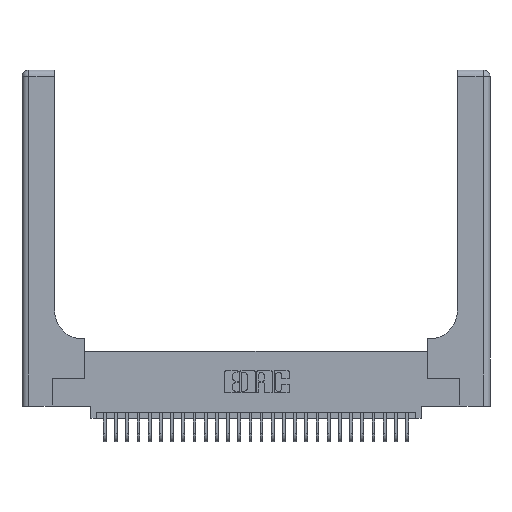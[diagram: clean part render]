
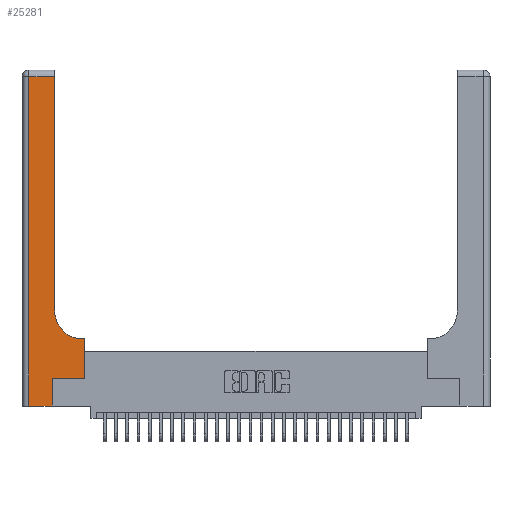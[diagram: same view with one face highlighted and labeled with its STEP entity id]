
A CAD part, top view. The second image highlights one B-rep face of the part: STEP entity #25281.
In plain terms, the highlighted planar face has unit normal (0, 0, 1).
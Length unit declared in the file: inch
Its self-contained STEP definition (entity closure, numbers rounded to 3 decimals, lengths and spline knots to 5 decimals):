
#190 = VECTOR ( 'NONE', #27991, 39.37008 ) ;
#392 = DIRECTION ( 'NONE',  ( -1., 0., 0. ) ) ;
#899 = VECTOR ( 'NONE', #27820, 39.37008 ) ;
#920 = LINE ( 'NONE', #17345, #13625 ) ;
#1758 = EDGE_CURVE ( 'NONE', #1877, #13865, #16058, .T. ) ;
#1764 = DIRECTION ( 'NONE',  ( 0., 0., -1. ) ) ;
#1877 = VERTEX_POINT ( 'NONE', #20327 ) ;
#2070 = EDGE_CURVE ( 'NONE', #19659, #1877, #29144, .T. ) ;
#2707 = CARTESIAN_POINT ( 'NONE',  ( 0.06, 0., 0.37 ) ) ;
#2768 = DIRECTION ( 'NONE',  ( 0., 1., 0. ) ) ;
#3035 = VECTOR ( 'NONE', #3798, 39.37008 ) ;
#3336 = CARTESIAN_POINT ( 'NONE',  ( 0.269, 0., 0.37 ) ) ;
#3798 = DIRECTION ( 'NONE',  ( 0., 1., 0. ) ) ;
#4294 = ORIENTED_EDGE ( 'NONE', *, *, #7521, .T. ) ;
#4740 = EDGE_CURVE ( 'NONE', #13865, #21605, #920, .T. ) ;
#6371 = ORIENTED_EDGE ( 'NONE', *, *, #29712, .T. ) ;
#6445 = CARTESIAN_POINT ( 'NONE',  ( 0.2915, 0.85, 0.37 ) ) ;
#6461 = EDGE_CURVE ( 'NONE', #21605, #19885, #23593, .T. ) ;
#7012 = CARTESIAN_POINT ( 'NONE',  ( 0.2915, 3., 0.37 ) ) ;
#7140 = CARTESIAN_POINT ( 'NONE',  ( 0.5585, 0.6, 0.37 ) ) ;
#7292 = EDGE_CURVE ( 'NONE', #17067, #9158, #20140, .T. ) ;
#7521 = EDGE_CURVE ( 'NONE', #14353, #17067, #23120, .T. ) ;
#7880 = VECTOR ( 'NONE', #2768, 39.37008 ) ;
#9158 = VERTEX_POINT ( 'NONE', #6445 ) ;
#9559 = ORIENTED_EDGE ( 'NONE', *, *, #6461, .T. ) ;
#10865 = ORIENTED_EDGE ( 'NONE', *, *, #13460, .T. ) ;
#11265 = CARTESIAN_POINT ( 'NONE',  ( 0.5415, 0.85, 0.37 ) ) ;
#11592 = CARTESIAN_POINT ( 'NONE',  ( 0.2915, 2.94, 0.37 ) ) ;
#13460 = EDGE_CURVE ( 'NONE', #25379, #14353, #15853, .T. ) ;
#13625 = VECTOR ( 'NONE', #21831, 39.37008 ) ;
#13744 = DIRECTION ( 'NONE',  ( -1., 0., 0. ) ) ;
#13865 = VERTEX_POINT ( 'NONE', #2707 ) ;
#13874 = DIRECTION ( 'NONE',  ( 1., 0., 0. ) ) ;
#13894 = ORIENTED_EDGE ( 'NONE', *, *, #7292, .T. ) ;
#14353 = VERTEX_POINT ( 'NONE', #7140 ) ;
#14548 = VECTOR ( 'NONE', #22116, 39.37008 ) ;
#15752 = AXIS2_PLACEMENT_3D ( 'NONE', #27879, #1764, #13744 ) ;
#15853 = LINE ( 'NONE', #20152, #899 ) ;
#16058 = LINE ( 'NONE', #24620, #14548 ) ;
#16567 = CARTESIAN_POINT ( 'NONE',  ( 0.5415, 0.6, 0.37 ) ) ;
#17067 = VERTEX_POINT ( 'NONE', #16567 ) ;
#17345 = CARTESIAN_POINT ( 'NONE',  ( 0., 0., 0.37 ) ) ;
#17773 = DIRECTION ( 'NONE',  ( -1., 0., 0. ) ) ;
#18026 = AXIS2_PLACEMENT_3D ( 'NONE', #11265, #23165, #13874 ) ;
#18626 = CARTESIAN_POINT ( 'NONE',  ( 0.5585, 0.25, 0.37 ) ) ;
#19452 = CARTESIAN_POINT ( 'NONE',  ( 0., 2.94, 0.37 ) ) ;
#19603 = CARTESIAN_POINT ( 'NONE',  ( 0.269, 0.25, 0.37 ) ) ;
#19659 = VERTEX_POINT ( 'NONE', #11592 ) ;
#19885 = VERTEX_POINT ( 'NONE', #19603 ) ;
#20140 = CIRCLE ( 'NONE', #18026, 0.25 ) ;
#20152 = CARTESIAN_POINT ( 'NONE',  ( 0.5585, 0.25, 0.37 ) ) ;
#20327 = CARTESIAN_POINT ( 'NONE',  ( 0.06, 2.94, 0.37 ) ) ;
#21017 = PLANE ( 'NONE',  #15752 ) ;
#21605 = VERTEX_POINT ( 'NONE', #3336 ) ;
#21831 = DIRECTION ( 'NONE',  ( 1., 0., 0. ) ) ;
#22116 = DIRECTION ( 'NONE',  ( 0., -1., 0. ) ) ;
#23120 = LINE ( 'NONE', #24380, #25346 ) ;
#23165 = DIRECTION ( 'NONE',  ( 0., 0., -1. ) ) ;
#23593 = LINE ( 'NONE', #26722, #7880 ) ;
#23782 = ORIENTED_EDGE ( 'NONE', *, *, #1758, .T. ) ;
#24380 = CARTESIAN_POINT ( 'NONE',  ( 0.2915, 0.6, 0.37 ) ) ;
#24620 = CARTESIAN_POINT ( 'NONE',  ( 0.06, 3., 0.37 ) ) ;
#25179 = LINE ( 'NONE', #25638, #190 ) ;
#25281 = ADVANCED_FACE ( 'NONE', ( #30031 ), #21017, .F. ) ;
#25346 = VECTOR ( 'NONE', #392, 39.37008 ) ;
#25379 = VERTEX_POINT ( 'NONE', #18626 ) ;
#25638 = CARTESIAN_POINT ( 'NONE',  ( 0.269, 0.25, 0.37 ) ) ;
#25833 = VECTOR ( 'NONE', #17773, 39.37008 ) ;
#26506 = LINE ( 'NONE', #7012, #3035 ) ;
#26722 = CARTESIAN_POINT ( 'NONE',  ( 0.269, 0., 0.37 ) ) ;
#27820 = DIRECTION ( 'NONE',  ( 0., 1., 0. ) ) ;
#27879 = CARTESIAN_POINT ( 'NONE',  ( 0., 3., 0.37 ) ) ;
#27991 = DIRECTION ( 'NONE',  ( 1., 0., 0. ) ) ;
#28536 = ORIENTED_EDGE ( 'NONE', *, *, #28564, .T. ) ;
#28564 = EDGE_CURVE ( 'NONE', #9158, #19659, #26506, .T. ) ;
#29144 = LINE ( 'NONE', #19452, #25833 ) ;
#29712 = EDGE_CURVE ( 'NONE', #19885, #25379, #25179, .T. ) ;
#30010 = ORIENTED_EDGE ( 'NONE', *, *, #2070, .T. ) ;
#30031 = FACE_OUTER_BOUND ( 'NONE', #30344, .T. ) ;
#30344 = EDGE_LOOP ( 'NONE', ( #28536, #30010, #23782, #30803, #9559, #6371, #10865, #4294, #13894 ) ) ;
#30803 = ORIENTED_EDGE ( 'NONE', *, *, #4740, .T. ) ;
